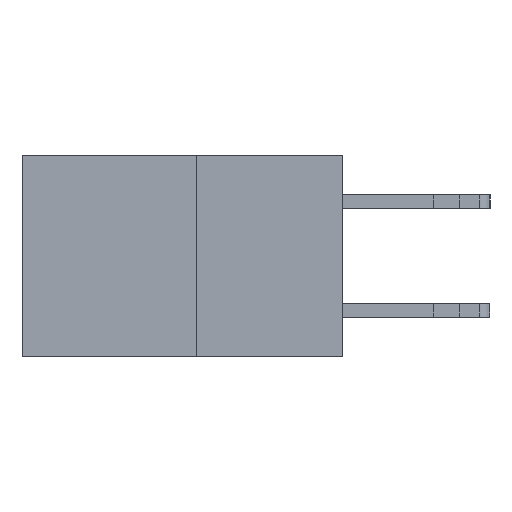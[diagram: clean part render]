
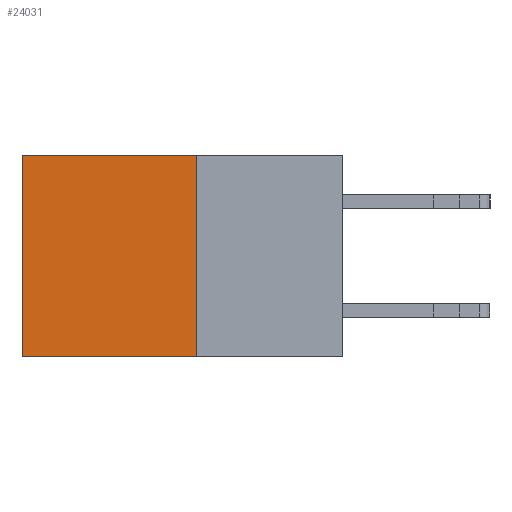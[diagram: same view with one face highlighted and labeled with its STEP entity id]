
A CAD part, left-side view. The second image highlights one B-rep face of the part: STEP entity #24031.
In plain terms, the highlighted planar face has unit normal (-1, 0, 0).
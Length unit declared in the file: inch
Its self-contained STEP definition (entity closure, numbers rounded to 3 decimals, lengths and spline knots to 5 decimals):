
#355 = DIRECTION ( 'NONE',  ( 0., 0., -1. ) ) ;
#383 = ORIENTED_EDGE ( 'NONE', *, *, #9522, .F. ) ;
#1633 = CARTESIAN_POINT ( 'NONE',  ( 0.277, 0.27, -0.37 ) ) ;
#2460 = ORIENTED_EDGE ( 'NONE', *, *, #5708, .T. ) ;
#2590 = LINE ( 'NONE', #22633, #11979 ) ;
#3481 = CARTESIAN_POINT ( 'NONE',  ( 0.277, 0.59, 0. ) ) ;
#3888 = DIRECTION ( 'NONE',  ( 0., 0., -1. ) ) ;
#5257 = EDGE_LOOP ( 'NONE', ( #18849, #383, #17895, #2460 ) ) ;
#5708 = EDGE_CURVE ( 'NONE', #12716, #15383, #2590, .T. ) ;
#6249 = CARTESIAN_POINT ( 'NONE',  ( 0.277, 0.59, -0.37 ) ) ;
#6775 = EDGE_CURVE ( 'NONE', #12716, #22260, #9760, .T. ) ;
#8369 = AXIS2_PLACEMENT_3D ( 'NONE', #13833, #15766, #3888 ) ;
#8932 = VECTOR ( 'NONE', #355, 39.37008 ) ;
#9340 = LINE ( 'NONE', #1633, #13348 ) ;
#9522 = EDGE_CURVE ( 'NONE', #22260, #10126, #9340, .T. ) ;
#9760 = LINE ( 'NONE', #11529, #14347 ) ;
#10126 = VERTEX_POINT ( 'NONE', #22686 ) ;
#10291 = FACE_OUTER_BOUND ( 'NONE', #5257, .T. ) ;
#11529 = CARTESIAN_POINT ( 'NONE',  ( 0.277, 0.27, -0.37 ) ) ;
#11600 = DIRECTION ( 'NONE',  ( 0., 1., 0. ) ) ;
#11882 = PLANE ( 'NONE',  #8369 ) ;
#11979 = VECTOR ( 'NONE', #22407, 39.37008 ) ;
#12716 = VERTEX_POINT ( 'NONE', #24527 ) ;
#13348 = VECTOR ( 'NONE', #11600, 39.37008 ) ;
#13833 = CARTESIAN_POINT ( 'NONE',  ( 0.277, 0.27, -0.37 ) ) ;
#14059 = DIRECTION ( 'NONE',  ( 0., 0., -1. ) ) ;
#14345 = EDGE_CURVE ( 'NONE', #15383, #10126, #23772, .T. ) ;
#14347 = VECTOR ( 'NONE', #14059, 39.37008 ) ;
#15383 = VERTEX_POINT ( 'NONE', #3481 ) ;
#15766 = DIRECTION ( 'NONE',  ( 1., 0., 0. ) ) ;
#16593 = CARTESIAN_POINT ( 'NONE',  ( 0.277, 0.27, -0.37 ) ) ;
#17895 = ORIENTED_EDGE ( 'NONE', *, *, #6775, .F. ) ;
#18849 = ORIENTED_EDGE ( 'NONE', *, *, #14345, .T. ) ;
#22260 = VERTEX_POINT ( 'NONE', #16593 ) ;
#22407 = DIRECTION ( 'NONE',  ( 0., 1., 0. ) ) ;
#22633 = CARTESIAN_POINT ( 'NONE',  ( 0.277, 0.27, 0. ) ) ;
#22686 = CARTESIAN_POINT ( 'NONE',  ( 0.277, 0.59, -0.37 ) ) ;
#23772 = LINE ( 'NONE', #6249, #8932 ) ;
#24031 = ADVANCED_FACE ( 'NONE', ( #10291 ), #11882, .F. ) ;
#24527 = CARTESIAN_POINT ( 'NONE',  ( 0.277, 0.27, 0. ) ) ;
